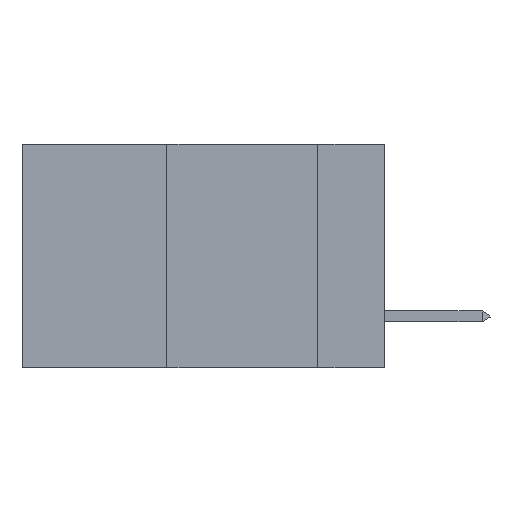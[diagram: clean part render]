
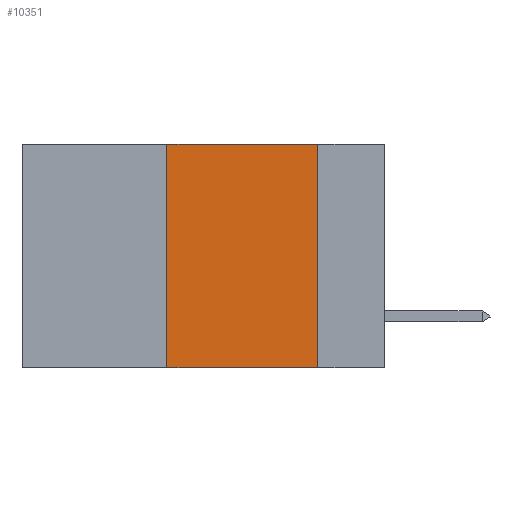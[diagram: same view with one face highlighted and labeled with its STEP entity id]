
A CAD part, left-side view. The second image highlights one B-rep face of the part: STEP entity #10351.
In plain terms, the highlighted planar face has unit normal (-1, 0, 0).
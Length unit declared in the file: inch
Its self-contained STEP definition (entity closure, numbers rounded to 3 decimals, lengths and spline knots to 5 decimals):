
#688 = DIRECTION ( 'NONE',  ( 0., 0., -1. ) ) ;
#840 = CARTESIAN_POINT ( 'NONE',  ( 0., 0.36, 0. ) ) ;
#1544 = CARTESIAN_POINT ( 'NONE',  ( 0., 0.36, -0.37 ) ) ;
#2794 = AXIS2_PLACEMENT_3D ( 'NONE', #5754, #10793, #8280 ) ;
#3211 = PLANE ( 'NONE',  #2794 ) ;
#3285 = FACE_OUTER_BOUND ( 'NONE', #9479, .T. ) ;
#3348 = VERTEX_POINT ( 'NONE', #6369 ) ;
#3405 = DIRECTION ( 'NONE',  ( 0., -1., 0. ) ) ;
#3692 = ORIENTED_EDGE ( 'NONE', *, *, #8044, .F. ) ;
#3902 = LINE ( 'NONE', #10665, #9543 ) ;
#4010 = EDGE_CURVE ( 'NONE', #10392, #3348, #10352, .T. ) ;
#4466 = VECTOR ( 'NONE', #6733, 39.37008 ) ;
#4913 = CARTESIAN_POINT ( 'NONE',  ( 0., 0.6, 0. ) ) ;
#4997 = CARTESIAN_POINT ( 'NONE',  ( 0., 0.11, -0.37 ) ) ;
#5256 = VECTOR ( 'NONE', #9869, 39.37008 ) ;
#5754 = CARTESIAN_POINT ( 'NONE',  ( 0., 0.6, 0. ) ) ;
#6141 = ORIENTED_EDGE ( 'NONE', *, *, #10823, .T. ) ;
#6369 = CARTESIAN_POINT ( 'NONE',  ( 0., 0.11, 0. ) ) ;
#6511 = CARTESIAN_POINT ( 'NONE',  ( 0., 0.6, -0.37 ) ) ;
#6573 = EDGE_CURVE ( 'NONE', #6866, #10392, #6724, .T. ) ;
#6724 = LINE ( 'NONE', #840, #4466 ) ;
#6733 = DIRECTION ( 'NONE',  ( 0., 0., 1. ) ) ;
#6866 = VERTEX_POINT ( 'NONE', #1544 ) ;
#7480 = CARTESIAN_POINT ( 'NONE',  ( 0., 0.36, 0. ) ) ;
#8044 = EDGE_CURVE ( 'NONE', #3348, #8200, #3902, .T. ) ;
#8152 = VECTOR ( 'NONE', #3405, 39.37008 ) ;
#8183 = ORIENTED_EDGE ( 'NONE', *, *, #4010, .F. ) ;
#8200 = VERTEX_POINT ( 'NONE', #4997 ) ;
#8280 = DIRECTION ( 'NONE',  ( 0., 0., -1. ) ) ;
#8676 = LINE ( 'NONE', #6511, #5256 ) ;
#9479 = EDGE_LOOP ( 'NONE', ( #3692, #8183, #9694, #6141 ) ) ;
#9543 = VECTOR ( 'NONE', #688, 39.37008 ) ;
#9694 = ORIENTED_EDGE ( 'NONE', *, *, #6573, .F. ) ;
#9869 = DIRECTION ( 'NONE',  ( 0., -1., 0. ) ) ;
#10351 = ADVANCED_FACE ( 'NONE', ( #3285 ), #3211, .F. ) ;
#10352 = LINE ( 'NONE', #4913, #8152 ) ;
#10392 = VERTEX_POINT ( 'NONE', #7480 ) ;
#10665 = CARTESIAN_POINT ( 'NONE',  ( 0., 0.11, 0. ) ) ;
#10793 = DIRECTION ( 'NONE',  ( 1., 0., 0. ) ) ;
#10823 = EDGE_CURVE ( 'NONE', #6866, #8200, #8676, .T. ) ;
